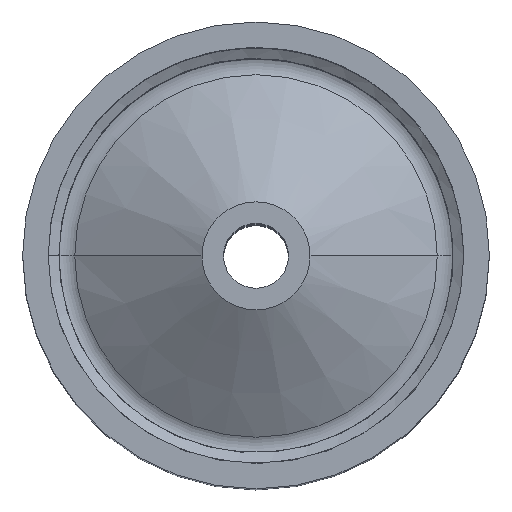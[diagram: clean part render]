
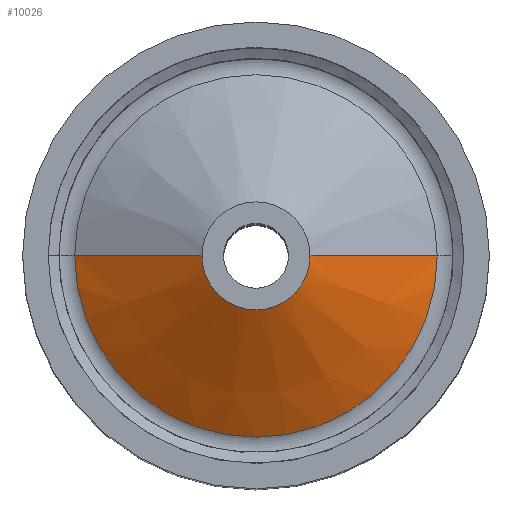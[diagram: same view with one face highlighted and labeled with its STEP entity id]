
A CAD part, top view. The second image highlights one B-rep face of the part: STEP entity #10026.
In plain terms, the highlighted conical face has half-angle 60 degrees and reference radius 22.384 mm.
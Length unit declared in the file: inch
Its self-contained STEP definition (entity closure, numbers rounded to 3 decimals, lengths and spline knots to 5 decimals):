
#378 = AXIS2_PLACEMENT_3D ( 'NONE', #4352, #1863, #2733 ) ;
#482 = DIRECTION ( 'NONE',  ( 0.866, 0., -0.5 ) ) ;
#559 = VECTOR ( 'NONE', #482, 39.37008 ) ;
#1305 = CARTESIAN_POINT ( 'NONE',  ( 0.88125, 0., 5.32735 ) ) ;
#1767 = LINE ( 'NONE', #1305, #559 ) ;
#1863 = DIRECTION ( 'NONE',  ( 0., 0., 1. ) ) ;
#1922 = VERTEX_POINT ( 'NONE', #7361 ) ;
#2039 = CIRCLE ( 'NONE', #378, 0.22901 ) ;
#2691 = CARTESIAN_POINT ( 'NONE',  ( 0., 0., 5.32735 ) ) ;
#2733 = DIRECTION ( 'NONE',  ( 1., 0., 0. ) ) ;
#2812 = CARTESIAN_POINT ( 'NONE',  ( 0., 0., 5.3923 ) ) ;
#3293 = AXIS2_PLACEMENT_3D ( 'NONE', #2691, #3638, #8794 ) ;
#3638 = DIRECTION ( 'NONE',  ( 0., 0., -1. ) ) ;
#4265 = ORIENTED_EDGE ( 'NONE', *, *, #4294, .F. ) ;
#4294 = EDGE_CURVE ( 'NONE', #5546, #8975, #2039, .T. ) ;
#4352 = CARTESIAN_POINT ( 'NONE',  ( 0., 0., 5.70392 ) ) ;
#4659 = AXIS2_PLACEMENT_3D ( 'NONE', #2812, #6371, #7116 ) ;
#5546 = VERTEX_POINT ( 'NONE', #8550 ) ;
#5729 = VERTEX_POINT ( 'NONE', #9573 ) ;
#5944 = LINE ( 'NONE', #7603, #7435 ) ;
#6371 = DIRECTION ( 'NONE',  ( 0., 0., 1. ) ) ;
#6710 = ORIENTED_EDGE ( 'NONE', *, *, #10353, .T. ) ;
#6753 = FACE_OUTER_BOUND ( 'NONE', #8745, .T. ) ;
#6886 = CONICAL_SURFACE ( 'NONE', #3293, 0.88125, 1.047 ) ;
#7116 = DIRECTION ( 'NONE',  ( -1., 0., 0. ) ) ;
#7361 = CARTESIAN_POINT ( 'NONE',  ( 0.76875, 0., 5.3923 ) ) ;
#7435 = VECTOR ( 'NONE', #9332, 39.37008 ) ;
#7603 = CARTESIAN_POINT ( 'NONE',  ( -0.88125, 0., 5.32735 ) ) ;
#7705 = CIRCLE ( 'NONE', #4659, 0.76875 ) ;
#8460 = EDGE_CURVE ( 'NONE', #8975, #1922, #1767, .T. ) ;
#8550 = CARTESIAN_POINT ( 'NONE',  ( -0.22901, 0., 5.70392 ) ) ;
#8745 = EDGE_LOOP ( 'NONE', ( #10503, #4265, #6710, #10021 ) ) ;
#8794 = DIRECTION ( 'NONE',  ( -1., 0., 0. ) ) ;
#8830 = EDGE_CURVE ( 'NONE', #5729, #1922, #7705, .T. ) ;
#8975 = VERTEX_POINT ( 'NONE', #9800 ) ;
#9332 = DIRECTION ( 'NONE',  ( -0.866, 0., -0.5 ) ) ;
#9573 = CARTESIAN_POINT ( 'NONE',  ( -0.76875, 0., 5.3923 ) ) ;
#9800 = CARTESIAN_POINT ( 'NONE',  ( 0.22901, 0., 5.70392 ) ) ;
#10021 = ORIENTED_EDGE ( 'NONE', *, *, #8830, .T. ) ;
#10026 = ADVANCED_FACE ( 'NONE', ( #6753 ), #6886, .T. ) ;
#10353 = EDGE_CURVE ( 'NONE', #5546, #5729, #5944, .T. ) ;
#10503 = ORIENTED_EDGE ( 'NONE', *, *, #8460, .F. ) ;
